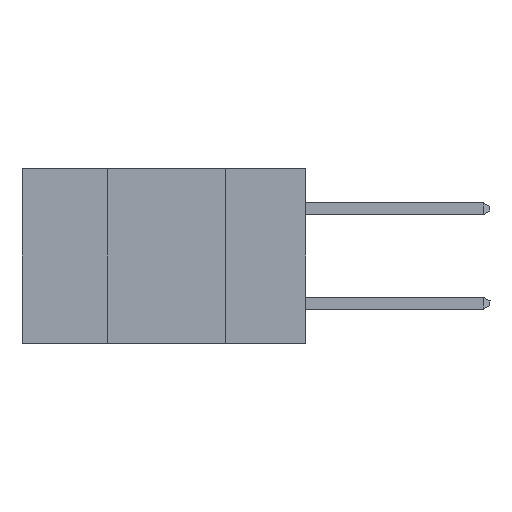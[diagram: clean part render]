
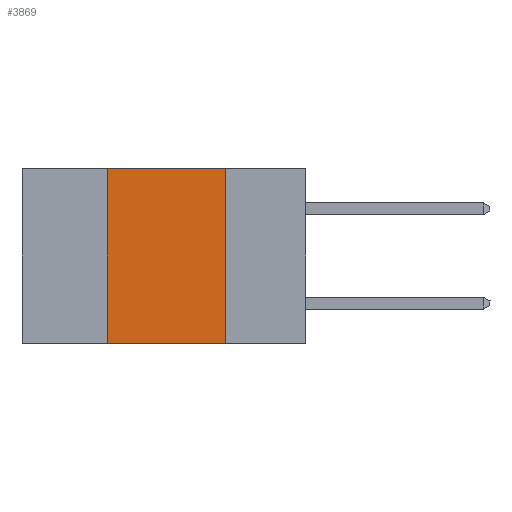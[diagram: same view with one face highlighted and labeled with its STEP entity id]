
A CAD part, left-side view. The second image highlights one B-rep face of the part: STEP entity #3869.
In plain terms, the highlighted planar face has unit normal (-1, 0, 0).
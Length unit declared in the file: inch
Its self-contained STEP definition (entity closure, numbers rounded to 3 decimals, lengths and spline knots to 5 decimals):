
#644 = CARTESIAN_POINT ( 'NONE',  ( 0., 0.6, 0. ) ) ;
#1574 = VERTEX_POINT ( 'NONE', #11071 ) ;
#1739 = FACE_OUTER_BOUND ( 'NONE', #6550, .T. ) ;
#1801 = AXIS2_PLACEMENT_3D ( 'NONE', #12229, #4719, #3534 ) ;
#2004 = CARTESIAN_POINT ( 'NONE',  ( 0., 0.17, 0. ) ) ;
#2332 = VECTOR ( 'NONE', #9993, 39.37008 ) ;
#2437 = ORIENTED_EDGE ( 'NONE', *, *, #10786, .T. ) ;
#2459 = CARTESIAN_POINT ( 'NONE',  ( 0., 0.6, -0.37 ) ) ;
#2553 = VERTEX_POINT ( 'NONE', #12160 ) ;
#2582 = LINE ( 'NONE', #9351, #6096 ) ;
#2615 = LINE ( 'NONE', #2459, #7663 ) ;
#2662 = LINE ( 'NONE', #644, #2332 ) ;
#3534 = DIRECTION ( 'NONE',  ( 0., 0., -1. ) ) ;
#3684 = PLANE ( 'NONE',  #1801 ) ;
#3869 = ADVANCED_FACE ( 'NONE', ( #1739 ), #3684, .F. ) ;
#4126 = DIRECTION ( 'NONE',  ( 0., 0., -1. ) ) ;
#4539 = VERTEX_POINT ( 'NONE', #4937 ) ;
#4719 = DIRECTION ( 'NONE',  ( 1., 0., 0. ) ) ;
#4937 = CARTESIAN_POINT ( 'NONE',  ( 0., 0.42, -0.37 ) ) ;
#5390 = ORIENTED_EDGE ( 'NONE', *, *, #5818, .F. ) ;
#5816 = EDGE_CURVE ( 'NONE', #7970, #2553, #8066, .T. ) ;
#5818 = EDGE_CURVE ( 'NONE', #4539, #1574, #2582, .T. ) ;
#6096 = VECTOR ( 'NONE', #10806, 39.37008 ) ;
#6550 = EDGE_LOOP ( 'NONE', ( #12619, #13495, #5390, #2437 ) ) ;
#6688 = DIRECTION ( 'NONE',  ( 0., -1., 0. ) ) ;
#7613 = EDGE_CURVE ( 'NONE', #1574, #7970, #2662, .T. ) ;
#7663 = VECTOR ( 'NONE', #6688, 39.37008 ) ;
#7970 = VERTEX_POINT ( 'NONE', #2004 ) ;
#8066 = LINE ( 'NONE', #8379, #10328 ) ;
#8379 = CARTESIAN_POINT ( 'NONE',  ( 0., 0.17, 0. ) ) ;
#9351 = CARTESIAN_POINT ( 'NONE',  ( 0., 0.42, 0. ) ) ;
#9993 = DIRECTION ( 'NONE',  ( 0., -1., 0. ) ) ;
#10328 = VECTOR ( 'NONE', #4126, 39.37008 ) ;
#10786 = EDGE_CURVE ( 'NONE', #4539, #2553, #2615, .T. ) ;
#10806 = DIRECTION ( 'NONE',  ( 0., 0., 1. ) ) ;
#11071 = CARTESIAN_POINT ( 'NONE',  ( 0., 0.42, 0. ) ) ;
#12160 = CARTESIAN_POINT ( 'NONE',  ( 0., 0.17, -0.37 ) ) ;
#12229 = CARTESIAN_POINT ( 'NONE',  ( 0., 0.6, 0. ) ) ;
#12619 = ORIENTED_EDGE ( 'NONE', *, *, #5816, .F. ) ;
#13495 = ORIENTED_EDGE ( 'NONE', *, *, #7613, .F. ) ;
